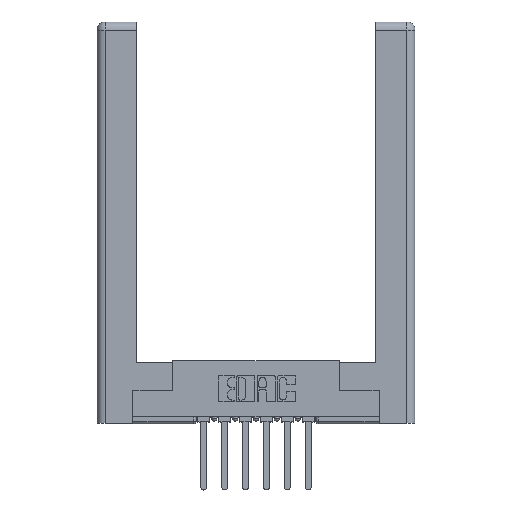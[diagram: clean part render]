
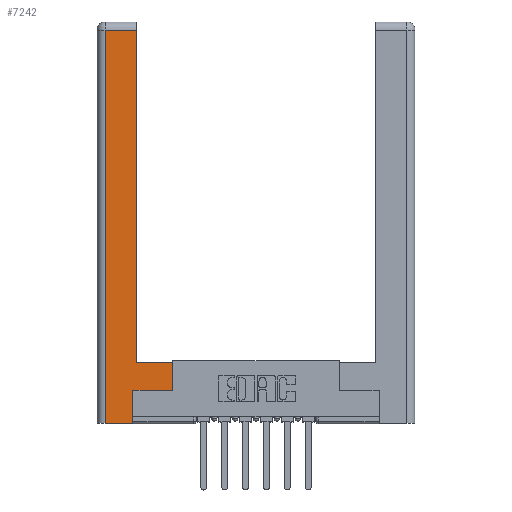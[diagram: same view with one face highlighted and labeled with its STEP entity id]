
A CAD part, top view. The second image highlights one B-rep face of the part: STEP entity #7242.
In plain terms, the highlighted planar face has unit normal (0, 0, 1).
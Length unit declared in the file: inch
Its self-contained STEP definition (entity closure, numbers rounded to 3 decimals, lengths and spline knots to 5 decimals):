
#213 = CARTESIAN_POINT ( 'NONE',  ( 0.295, 0.45, 0. ) ) ;
#302 = VECTOR ( 'NONE', #6309, 39.37008 ) ;
#341 = LINE ( 'NONE', #6571, #6141 ) ;
#490 = ORIENTED_EDGE ( 'NONE', *, *, #3734, .T. ) ;
#515 = LINE ( 'NONE', #9696, #6475 ) ;
#596 = VERTEX_POINT ( 'NONE', #3091 ) ;
#616 = CARTESIAN_POINT ( 'NONE',  ( 0.295, 2.94, 0. ) ) ;
#642 = ORIENTED_EDGE ( 'NONE', *, *, #12591, .T. ) ;
#684 = DIRECTION ( 'NONE',  ( 0., 1., 0. ) ) ;
#812 = EDGE_CURVE ( 'NONE', #2935, #3398, #5553, .T. ) ;
#1341 = FACE_OUTER_BOUND ( 'NONE', #8574, .T. ) ;
#1779 = EDGE_CURVE ( 'NONE', #6553, #6260, #515, .T. ) ;
#1835 = PLANE ( 'NONE',  #4520 ) ;
#2080 = CARTESIAN_POINT ( 'NONE',  ( 0.0615, 0., 0. ) ) ;
#2316 = VERTEX_POINT ( 'NONE', #2080 ) ;
#2374 = EDGE_CURVE ( 'NONE', #596, #2316, #7713, .T. ) ;
#2672 = CARTESIAN_POINT ( 'NONE',  ( 0.565, 0.245, 0. ) ) ;
#2679 = VECTOR ( 'NONE', #11851, 39.37008 ) ;
#2935 = VERTEX_POINT ( 'NONE', #11811 ) ;
#3091 = CARTESIAN_POINT ( 'NONE',  ( 0.0615, 2.94, 0. ) ) ;
#3384 = VERTEX_POINT ( 'NONE', #616 ) ;
#3398 = VERTEX_POINT ( 'NONE', #10766 ) ;
#3734 = EDGE_CURVE ( 'NONE', #3384, #596, #11101, .T. ) ;
#3812 = DIRECTION ( 'NONE',  ( 0., 0., -1. ) ) ;
#4351 = ORIENTED_EDGE ( 'NONE', *, *, #812, .T. ) ;
#4356 = DIRECTION ( 'NONE',  ( 0., 1., 0. ) ) ;
#4520 = AXIS2_PLACEMENT_3D ( 'NONE', #9801, #3812, #7926 ) ;
#5140 = ORIENTED_EDGE ( 'NONE', *, *, #5735, .T. ) ;
#5386 = CARTESIAN_POINT ( 'NONE',  ( 0.0615, 0., 0. ) ) ;
#5501 = CARTESIAN_POINT ( 'NONE',  ( 0.265, 0.245, 0. ) ) ;
#5553 = LINE ( 'NONE', #2672, #9468 ) ;
#5691 = LINE ( 'NONE', #11823, #11456 ) ;
#5735 = EDGE_CURVE ( 'NONE', #2316, #9654, #7505, .T. ) ;
#6141 = VECTOR ( 'NONE', #9531, 39.37008 ) ;
#6260 = VERTEX_POINT ( 'NONE', #213 ) ;
#6309 = DIRECTION ( 'NONE',  ( 1., 0., 0. ) ) ;
#6334 = LINE ( 'NONE', #5501, #6480 ) ;
#6475 = VECTOR ( 'NONE', #10608, 39.37008 ) ;
#6480 = VECTOR ( 'NONE', #4356, 39.37008 ) ;
#6553 = VERTEX_POINT ( 'NONE', #6847 ) ;
#6571 = CARTESIAN_POINT ( 'NONE',  ( 0.295, 3., 0. ) ) ;
#6847 = CARTESIAN_POINT ( 'NONE',  ( 0.565, 0.45, 0. ) ) ;
#7242 = ADVANCED_FACE ( 'NONE', ( #1341 ), #1835, .F. ) ;
#7284 = DIRECTION ( 'NONE',  ( 0., -1., 0. ) ) ;
#7466 = ORIENTED_EDGE ( 'NONE', *, *, #9010, .T. ) ;
#7505 = LINE ( 'NONE', #10367, #302 ) ;
#7658 = ORIENTED_EDGE ( 'NONE', *, *, #1779, .T. ) ;
#7713 = LINE ( 'NONE', #5386, #11422 ) ;
#7718 = DIRECTION ( 'NONE',  ( 1., 0., 0. ) ) ;
#7784 = CARTESIAN_POINT ( 'NONE',  ( 0.0615, 2.94, 0. ) ) ;
#7926 = DIRECTION ( 'NONE',  ( -1., 0., 0. ) ) ;
#8326 = CARTESIAN_POINT ( 'NONE',  ( 0.265, 0., 0. ) ) ;
#8574 = EDGE_LOOP ( 'NONE', ( #10458, #490, #11204, #5140, #7466, #4351, #642, #7658 ) ) ;
#9010 = EDGE_CURVE ( 'NONE', #9654, #2935, #6334, .T. ) ;
#9468 = VECTOR ( 'NONE', #7718, 39.37008 ) ;
#9531 = DIRECTION ( 'NONE',  ( 0., 1., 0. ) ) ;
#9654 = VERTEX_POINT ( 'NONE', #8326 ) ;
#9696 = CARTESIAN_POINT ( 'NONE',  ( 0.295, 0.45, 0. ) ) ;
#9801 = CARTESIAN_POINT ( 'NONE',  ( 0., 0., 0. ) ) ;
#10367 = CARTESIAN_POINT ( 'NONE',  ( 0.265, 0., 0. ) ) ;
#10422 = EDGE_CURVE ( 'NONE', #6260, #3384, #341, .T. ) ;
#10458 = ORIENTED_EDGE ( 'NONE', *, *, #10422, .T. ) ;
#10608 = DIRECTION ( 'NONE',  ( -1., 0., 0. ) ) ;
#10766 = CARTESIAN_POINT ( 'NONE',  ( 0.565, 0.245, 0. ) ) ;
#11101 = LINE ( 'NONE', #7784, #2679 ) ;
#11204 = ORIENTED_EDGE ( 'NONE', *, *, #2374, .T. ) ;
#11422 = VECTOR ( 'NONE', #7284, 39.37008 ) ;
#11456 = VECTOR ( 'NONE', #684, 39.37008 ) ;
#11811 = CARTESIAN_POINT ( 'NONE',  ( 0.265, 0.245, 0. ) ) ;
#11823 = CARTESIAN_POINT ( 'NONE',  ( 0.565, 0.45, 0. ) ) ;
#11851 = DIRECTION ( 'NONE',  ( -1., 0., 0. ) ) ;
#12591 = EDGE_CURVE ( 'NONE', #3398, #6553, #5691, .T. ) ;
